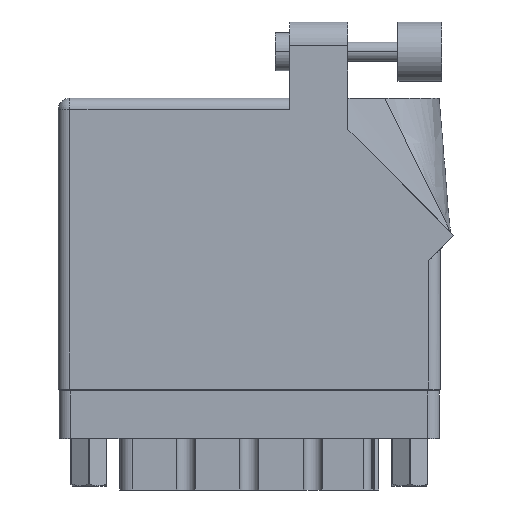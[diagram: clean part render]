
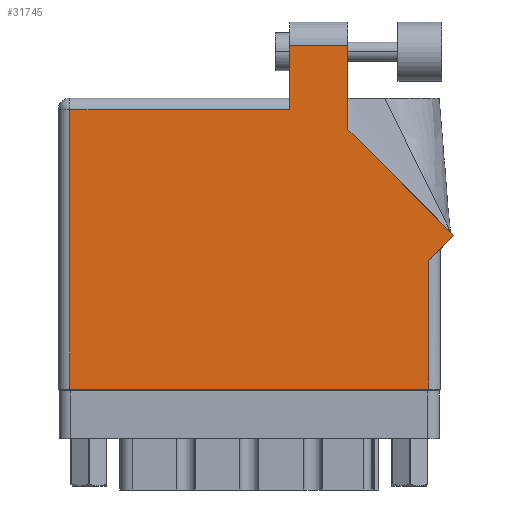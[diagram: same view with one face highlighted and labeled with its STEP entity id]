
A CAD part, front view. The second image highlights one B-rep face of the part: STEP entity #31745.
In plain terms, the highlighted face is planar.
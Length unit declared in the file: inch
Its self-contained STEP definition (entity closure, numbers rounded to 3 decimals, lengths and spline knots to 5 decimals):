
#254 = CARTESIAN_POINT ( 'NONE',  ( 1.524, 1.36442, 0. ) ) ;
#358 = VECTOR ( 'NONE', #15003, 39.37008 ) ;
#918 = ORIENTED_EDGE ( 'NONE', *, *, #9963, .T. ) ;
#1685 = VECTOR ( 'NONE', #42844, 39.37008 ) ;
#2464 = CARTESIAN_POINT ( 'NONE',  ( 1.217, 1.805, 0. ) ) ;
#2968 = VERTEX_POINT ( 'NONE', #38062 ) ;
#3330 = DIRECTION ( 'NONE',  ( -1., 0., 0. ) ) ;
#3837 = DIRECTION ( 'NONE',  ( 0., 1., 0. ) ) ;
#3878 = VERTEX_POINT ( 'NONE', #10379 ) ;
#6512 = VERTEX_POINT ( 'NONE', #35309 ) ;
#6628 = CARTESIAN_POINT ( 'NONE',  ( 1.217, 1.53, 0. ) ) ;
#7087 = LINE ( 'NONE', #42481, #40276 ) ;
#7753 = ORIENTED_EDGE ( 'NONE', *, *, #25000, .T. ) ;
#7776 = CARTESIAN_POINT ( 'NONE',  ( 1.524, 1.36442, 0. ) ) ;
#7844 = VERTEX_POINT ( 'NONE', #2464 ) ;
#8109 = CARTESIAN_POINT ( 'NONE',  ( 0., 1.468, 0. ) ) ;
#8690 = EDGE_CURVE ( 'NONE', #2968, #6512, #11440, .T. ) ;
#8960 = LINE ( 'NONE', #19695, #1685 ) ;
#9593 = EDGE_CURVE ( 'NONE', #49478, #42129, #8960, .T. ) ;
#9705 = VECTOR ( 'NONE', #14081, 39.37008 ) ;
#9963 = EDGE_CURVE ( 'NONE', #3878, #49478, #7087, .T. ) ;
#10041 = ORIENTED_EDGE ( 'NONE', *, *, #24741, .T. ) ;
#10379 = CARTESIAN_POINT ( 'NONE',  ( 0.062, 0., 0. ) ) ;
#10954 = EDGE_LOOP ( 'NONE', ( #21316, #42506, #39893, #34392, #30271, #918, #34258, #10041, #7753 ) ) ;
#11440 = LINE ( 'NONE', #8109, #40963 ) ;
#11809 = LINE ( 'NONE', #28478, #31082 ) ;
#12870 = AXIS2_PLACEMENT_3D ( 'NONE', #43220, #47096, #27943 ) ;
#13943 = LINE ( 'NONE', #38038, #23035 ) ;
#14081 = DIRECTION ( 'NONE',  ( 0., -1., 0. ) ) ;
#15003 = DIRECTION ( 'NONE',  ( 0., -1., 0. ) ) ;
#17320 = VECTOR ( 'NONE', #19133, 39.37008 ) ;
#17974 = LINE ( 'NONE', #38420, #17320 ) ;
#19133 = DIRECTION ( 'NONE',  ( 0.707, 0.707, 0. ) ) ;
#19695 = CARTESIAN_POINT ( 'NONE',  ( 1.948, 0.737, 0. ) ) ;
#19775 = DIRECTION ( 'NONE',  ( -1., 0., 0. ) ) ;
#21316 = ORIENTED_EDGE ( 'NONE', *, *, #43197, .T. ) ;
#23035 = VECTOR ( 'NONE', #3330, 39.37008 ) ;
#23403 = PLANE ( 'NONE',  #12870 ) ;
#24061 = CARTESIAN_POINT ( 'NONE',  ( 1.948, 0.675, 0. ) ) ;
#24741 = EDGE_CURVE ( 'NONE', #42129, #39941, #17974, .T. ) ;
#25000 = EDGE_CURVE ( 'NONE', #39941, #26875, #11809, .T. ) ;
#26875 = VERTEX_POINT ( 'NONE', #7776 ) ;
#27943 = DIRECTION ( 'NONE',  ( -1., 0., 0. ) ) ;
#28478 = CARTESIAN_POINT ( 'NONE',  ( 2.08071, 0.80771, 0. ) ) ;
#29700 = CARTESIAN_POINT ( 'NONE',  ( 1.948, 0., 0. ) ) ;
#30068 = VERTEX_POINT ( 'NONE', #30531 ) ;
#30271 = ORIENTED_EDGE ( 'NONE', *, *, #39424, .T. ) ;
#30531 = CARTESIAN_POINT ( 'NONE',  ( 1.524, 1.805, 0. ) ) ;
#31082 = VECTOR ( 'NONE', #32364, 39.37008 ) ;
#31745 = ADVANCED_FACE ( 'NONE', ( #48227 ), #23403, .F. ) ;
#32364 = DIRECTION ( 'NONE',  ( -0.707, 0.707, 0. ) ) ;
#34168 = LINE ( 'NONE', #34183, #358 ) ;
#34183 = CARTESIAN_POINT ( 'NONE',  ( 0.062, 0., 0. ) ) ;
#34258 = ORIENTED_EDGE ( 'NONE', *, *, #9593, .T. ) ;
#34392 = ORIENTED_EDGE ( 'NONE', *, *, #8690, .T. ) ;
#35309 = CARTESIAN_POINT ( 'NONE',  ( 0.062, 1.468, 0. ) ) ;
#36995 = EDGE_CURVE ( 'NONE', #30068, #7844, #13943, .T. ) ;
#38038 = CARTESIAN_POINT ( 'NONE',  ( 1.217, 1.805, 0. ) ) ;
#38062 = CARTESIAN_POINT ( 'NONE',  ( 1.217, 1.468, 0. ) ) ;
#38420 = CARTESIAN_POINT ( 'NONE',  ( 2.01, 0.737, 0. ) ) ;
#39424 = EDGE_CURVE ( 'NONE', #6512, #3878, #34168, .T. ) ;
#39893 = ORIENTED_EDGE ( 'NONE', *, *, #47381, .T. ) ;
#39941 = VERTEX_POINT ( 'NONE', #44885 ) ;
#40276 = VECTOR ( 'NONE', #49876, 39.37008 ) ;
#40757 = VECTOR ( 'NONE', #3837, 39.37008 ) ;
#40963 = VECTOR ( 'NONE', #19775, 39.37008 ) ;
#41617 = LINE ( 'NONE', #6628, #9705 ) ;
#42129 = VERTEX_POINT ( 'NONE', #24061 ) ;
#42481 = CARTESIAN_POINT ( 'NONE',  ( 0., 0., 0. ) ) ;
#42506 = ORIENTED_EDGE ( 'NONE', *, *, #36995, .T. ) ;
#42844 = DIRECTION ( 'NONE',  ( 0., 1., 0. ) ) ;
#43197 = EDGE_CURVE ( 'NONE', #26875, #30068, #46756, .T. ) ;
#43220 = CARTESIAN_POINT ( 'NONE',  ( 0., 1.53, 0. ) ) ;
#44885 = CARTESIAN_POINT ( 'NONE',  ( 2.08071, 0.80771, 0. ) ) ;
#46756 = LINE ( 'NONE', #254, #40757 ) ;
#47096 = DIRECTION ( 'NONE',  ( 0., 0., -1. ) ) ;
#47381 = EDGE_CURVE ( 'NONE', #7844, #2968, #41617, .T. ) ;
#48227 = FACE_OUTER_BOUND ( 'NONE', #10954, .T. ) ;
#49478 = VERTEX_POINT ( 'NONE', #29700 ) ;
#49876 = DIRECTION ( 'NONE',  ( 1., 0., 0. ) ) ;
